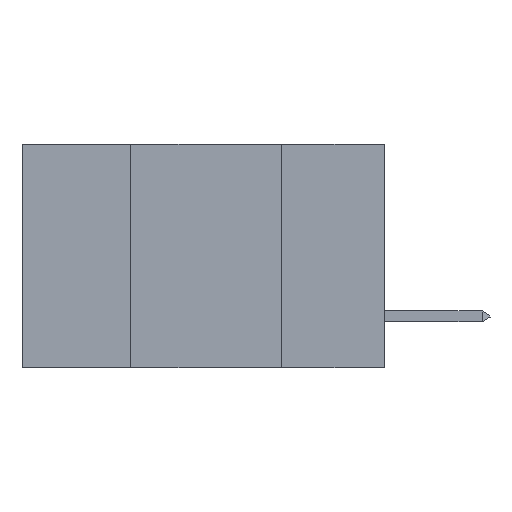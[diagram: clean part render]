
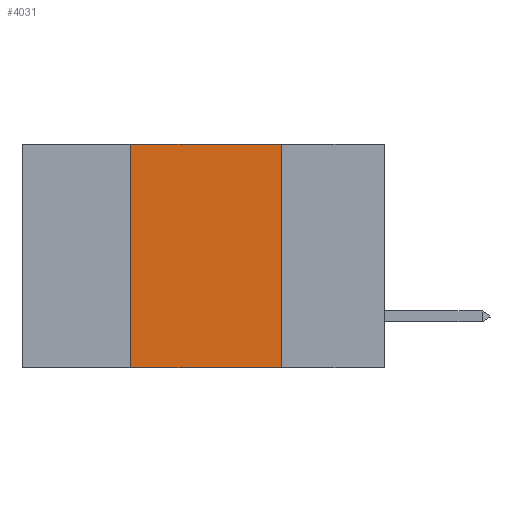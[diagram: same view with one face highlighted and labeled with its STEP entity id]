
A CAD part, left-side view. The second image highlights one B-rep face of the part: STEP entity #4031.
In plain terms, the highlighted planar face has unit normal (-1, 0, 0).
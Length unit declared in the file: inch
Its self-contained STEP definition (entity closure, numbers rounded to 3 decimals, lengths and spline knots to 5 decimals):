
#745 = LINE ( 'NONE', #11404, #9856 ) ;
#2376 = CARTESIAN_POINT ( 'NONE',  ( 0., 0.17, 0. ) ) ;
#2585 = EDGE_CURVE ( 'NONE', #13945, #11129, #17994, .T. ) ;
#2753 = ORIENTED_EDGE ( 'NONE', *, *, #10233, .F. ) ;
#4031 = ADVANCED_FACE ( 'NONE', ( #17694 ), #13462, .F. ) ;
#4363 = VECTOR ( 'NONE', #12913, 39.37008 ) ;
#4686 = CARTESIAN_POINT ( 'NONE',  ( 0., 0.42, 0. ) ) ;
#4711 = CARTESIAN_POINT ( 'NONE',  ( 0., 0.6, 0. ) ) ;
#5012 = EDGE_CURVE ( 'NONE', #15938, #8084, #8249, .T. ) ;
#5143 = LINE ( 'NONE', #15736, #16299 ) ;
#5651 = CARTESIAN_POINT ( 'NONE',  ( 0., 0.17, -0.37 ) ) ;
#5994 = CARTESIAN_POINT ( 'NONE',  ( 0., 0.42, 0. ) ) ;
#6201 = DIRECTION ( 'NONE',  ( 0., 0., -1. ) ) ;
#6389 = VECTOR ( 'NONE', #10144, 39.37008 ) ;
#7507 = ORIENTED_EDGE ( 'NONE', *, *, #5012, .F. ) ;
#8084 = VERTEX_POINT ( 'NONE', #5651 ) ;
#8249 = LINE ( 'NONE', #18710, #4363 ) ;
#9856 = VECTOR ( 'NONE', #9935, 39.37008 ) ;
#9935 = DIRECTION ( 'NONE',  ( 0., -1., 0. ) ) ;
#10144 = DIRECTION ( 'NONE',  ( 0., 0., 1. ) ) ;
#10233 = EDGE_CURVE ( 'NONE', #11129, #15938, #745, .T. ) ;
#11129 = VERTEX_POINT ( 'NONE', #4686 ) ;
#11404 = CARTESIAN_POINT ( 'NONE',  ( 0., 0.6, 0. ) ) ;
#11407 = DIRECTION ( 'NONE',  ( 0., -1., 0. ) ) ;
#12913 = DIRECTION ( 'NONE',  ( 0., 0., -1. ) ) ;
#13462 = PLANE ( 'NONE',  #15674 ) ;
#13850 = EDGE_CURVE ( 'NONE', #13945, #8084, #5143, .T. ) ;
#13945 = VERTEX_POINT ( 'NONE', #18265 ) ;
#14031 = EDGE_LOOP ( 'NONE', ( #7507, #2753, #17378, #17075 ) ) ;
#14919 = DIRECTION ( 'NONE',  ( 1., 0., 0. ) ) ;
#15674 = AXIS2_PLACEMENT_3D ( 'NONE', #4711, #14919, #6201 ) ;
#15736 = CARTESIAN_POINT ( 'NONE',  ( 0., 0.6, -0.37 ) ) ;
#15938 = VERTEX_POINT ( 'NONE', #2376 ) ;
#16299 = VECTOR ( 'NONE', #11407, 39.37008 ) ;
#17075 = ORIENTED_EDGE ( 'NONE', *, *, #13850, .T. ) ;
#17378 = ORIENTED_EDGE ( 'NONE', *, *, #2585, .F. ) ;
#17694 = FACE_OUTER_BOUND ( 'NONE', #14031, .T. ) ;
#17994 = LINE ( 'NONE', #5994, #6389 ) ;
#18265 = CARTESIAN_POINT ( 'NONE',  ( 0., 0.42, -0.37 ) ) ;
#18710 = CARTESIAN_POINT ( 'NONE',  ( 0., 0.17, 0. ) ) ;
